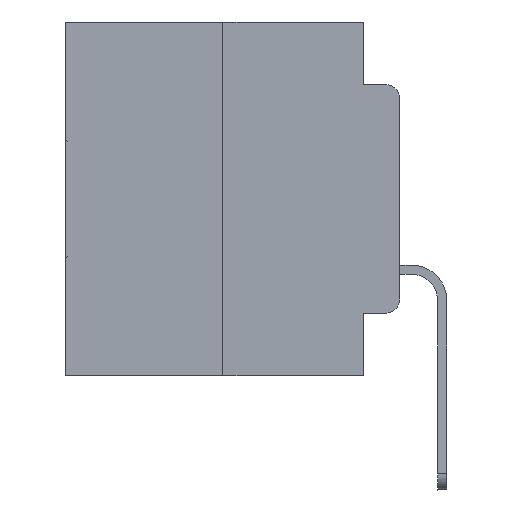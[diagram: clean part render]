
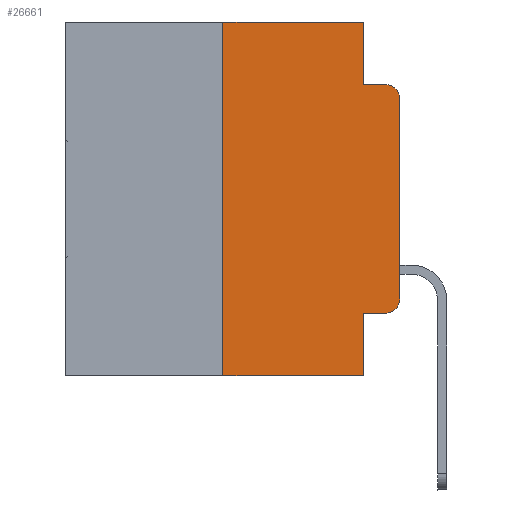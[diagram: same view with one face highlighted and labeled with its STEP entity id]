
A CAD part, left-side view. The second image highlights one B-rep face of the part: STEP entity #26661.
In plain terms, the highlighted planar face has unit normal (-1, 0, 0).
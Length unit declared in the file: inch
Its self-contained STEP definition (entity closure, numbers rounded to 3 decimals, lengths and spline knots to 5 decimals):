
#700 = LINE ( 'NONE', #10163, #25883 ) ;
#1578 = AXIS2_PLACEMENT_3D ( 'NONE', #21687, #19666, #24629 ) ;
#1926 = VERTEX_POINT ( 'NONE', #29517 ) ;
#1972 = VERTEX_POINT ( 'NONE', #27355 ) ;
#2471 = ORIENTED_EDGE ( 'NONE', *, *, #15398, .T. ) ;
#2717 = VECTOR ( 'NONE', #21556, 39.37008 ) ;
#2734 = VECTOR ( 'NONE', #13580, 39.37008 ) ;
#2752 = CARTESIAN_POINT ( 'NONE',  ( 0., 0.051, 0. ) ) ;
#2948 = EDGE_CURVE ( 'NONE', #13818, #6279, #14634, .T. ) ;
#3009 = DIRECTION ( 'NONE',  ( 0., -1., 0. ) ) ;
#3579 = CARTESIAN_POINT ( 'NONE',  ( 0., 0.473, 0. ) ) ;
#3864 = CARTESIAN_POINT ( 'NONE',  ( 0., 0., -0.1085 ) ) ;
#4123 = DIRECTION ( 'NONE',  ( 0., 0., 1. ) ) ;
#4128 = LINE ( 'NONE', #30042, #2734 ) ;
#4131 = ORIENTED_EDGE ( 'NONE', *, *, #2948, .F. ) ;
#4322 = VERTEX_POINT ( 'NONE', #20371 ) ;
#5908 = CARTESIAN_POINT ( 'NONE',  ( 0., 0.051, -0.0885 ) ) ;
#6057 = CARTESIAN_POINT ( 'NONE',  ( 0., 0.02, -0.4115 ) ) ;
#6279 = VERTEX_POINT ( 'NONE', #26697 ) ;
#7199 = EDGE_LOOP ( 'NONE', ( #2471, #22562, #4131, #20885, #15240, #29669, #28147, #19175, #14869, #29371 ) ) ;
#7861 = CIRCLE ( 'NONE', #21219, 0.02 ) ;
#8037 = CARTESIAN_POINT ( 'NONE',  ( 0., 0.051, 0. ) ) ;
#8534 = DIRECTION ( 'NONE',  ( 0., 0., -1. ) ) ;
#8654 = CARTESIAN_POINT ( 'NONE',  ( 0., 0.473, -0.5 ) ) ;
#8735 = EDGE_CURVE ( 'NONE', #27300, #13270, #7861, .T. ) ;
#9393 = EDGE_CURVE ( 'NONE', #30170, #6279, #29191, .T. ) ;
#9553 = CARTESIAN_POINT ( 'NONE',  ( 0., 0.051, -0.0885 ) ) ;
#10163 = CARTESIAN_POINT ( 'NONE',  ( 0., 0.051, 0. ) ) ;
#10689 = DIRECTION ( 'NONE',  ( 0., 0., -1. ) ) ;
#11706 = VECTOR ( 'NONE', #27333, 39.37008 ) ;
#11809 = DIRECTION ( 'NONE',  ( -1., 0., 0. ) ) ;
#12364 = FACE_OUTER_BOUND ( 'NONE', #7199, .T. ) ;
#12744 = EDGE_CURVE ( 'NONE', #4322, #21871, #700, .T. ) ;
#13270 = VERTEX_POINT ( 'NONE', #15978 ) ;
#13580 = DIRECTION ( 'NONE',  ( 0., 0., 1. ) ) ;
#13818 = VERTEX_POINT ( 'NONE', #9553 ) ;
#14634 = LINE ( 'NONE', #5908, #16709 ) ;
#14678 = CARTESIAN_POINT ( 'NONE',  ( 0., 0.051, -0.5 ) ) ;
#14724 = LINE ( 'NONE', #23723, #2717 ) ;
#14869 = ORIENTED_EDGE ( 'NONE', *, *, #29958, .T. ) ;
#15240 = ORIENTED_EDGE ( 'NONE', *, *, #20910, .F. ) ;
#15398 = EDGE_CURVE ( 'NONE', #13270, #30170, #4128, .T. ) ;
#15481 = LINE ( 'NONE', #8654, #21577 ) ;
#15808 = AXIS2_PLACEMENT_3D ( 'NONE', #18562, #27743, #17965 ) ;
#15978 = CARTESIAN_POINT ( 'NONE',  ( 0., 0., -0.3915 ) ) ;
#16583 = VECTOR ( 'NONE', #10689, 39.37008 ) ;
#16709 = VECTOR ( 'NONE', #3009, 39.37008 ) ;
#17965 = DIRECTION ( 'NONE',  ( 0., 0., -1. ) ) ;
#18332 = VERTEX_POINT ( 'NONE', #2752 ) ;
#18562 = CARTESIAN_POINT ( 'NONE',  ( 0., 0.02, -0.1085 ) ) ;
#18685 = LINE ( 'NONE', #28161, #27890 ) ;
#19175 = ORIENTED_EDGE ( 'NONE', *, *, #12744, .F. ) ;
#19666 = DIRECTION ( 'NONE',  ( 1., 0., 0. ) ) ;
#20180 = EDGE_CURVE ( 'NONE', #1926, #21871, #15481, .T. ) ;
#20371 = CARTESIAN_POINT ( 'NONE',  ( 0., 0.051, -0.4115 ) ) ;
#20885 = ORIENTED_EDGE ( 'NONE', *, *, #30093, .F. ) ;
#20910 = EDGE_CURVE ( 'NONE', #1972, #18332, #21619, .T. ) ;
#21219 = AXIS2_PLACEMENT_3D ( 'NONE', #26714, #11809, #8534 ) ;
#21556 = DIRECTION ( 'NONE',  ( 0., -1., 0. ) ) ;
#21577 = VECTOR ( 'NONE', #29611, 39.37008 ) ;
#21619 = LINE ( 'NONE', #3579, #11706 ) ;
#21687 = CARTESIAN_POINT ( 'NONE',  ( 0., 0.473, 0. ) ) ;
#21871 = VERTEX_POINT ( 'NONE', #14678 ) ;
#22562 = ORIENTED_EDGE ( 'NONE', *, *, #9393, .T. ) ;
#23723 = CARTESIAN_POINT ( 'NONE',  ( 0., 0.051, -0.4115 ) ) ;
#24469 = PLANE ( 'NONE',  #1578 ) ;
#24629 = DIRECTION ( 'NONE',  ( 0., 0., -1. ) ) ;
#24955 = LINE ( 'NONE', #8037, #16583 ) ;
#25883 = VECTOR ( 'NONE', #29111, 39.37008 ) ;
#26661 = ADVANCED_FACE ( 'NONE', ( #12364 ), #24469, .F. ) ;
#26697 = CARTESIAN_POINT ( 'NONE',  ( 0., 0.02, -0.0885 ) ) ;
#26714 = CARTESIAN_POINT ( 'NONE',  ( 0., 0.02, -0.3915 ) ) ;
#27300 = VERTEX_POINT ( 'NONE', #6057 ) ;
#27333 = DIRECTION ( 'NONE',  ( 0., -1., 0. ) ) ;
#27355 = CARTESIAN_POINT ( 'NONE',  ( 0., 0.25, 0. ) ) ;
#27743 = DIRECTION ( 'NONE',  ( -1., 0., 0. ) ) ;
#27890 = VECTOR ( 'NONE', #4123, 39.37008 ) ;
#27910 = EDGE_CURVE ( 'NONE', #1926, #1972, #18685, .T. ) ;
#28147 = ORIENTED_EDGE ( 'NONE', *, *, #20180, .T. ) ;
#28161 = CARTESIAN_POINT ( 'NONE',  ( 0., 0.25, 0. ) ) ;
#29111 = DIRECTION ( 'NONE',  ( 0., 0., -1. ) ) ;
#29191 = CIRCLE ( 'NONE', #15808, 0.02 ) ;
#29371 = ORIENTED_EDGE ( 'NONE', *, *, #8735, .T. ) ;
#29517 = CARTESIAN_POINT ( 'NONE',  ( 0., 0.25, -0.5 ) ) ;
#29611 = DIRECTION ( 'NONE',  ( 0., -1., 0. ) ) ;
#29669 = ORIENTED_EDGE ( 'NONE', *, *, #27910, .F. ) ;
#29958 = EDGE_CURVE ( 'NONE', #4322, #27300, #14724, .T. ) ;
#30042 = CARTESIAN_POINT ( 'NONE',  ( 0., 0., 0. ) ) ;
#30093 = EDGE_CURVE ( 'NONE', #18332, #13818, #24955, .T. ) ;
#30170 = VERTEX_POINT ( 'NONE', #3864 ) ;
